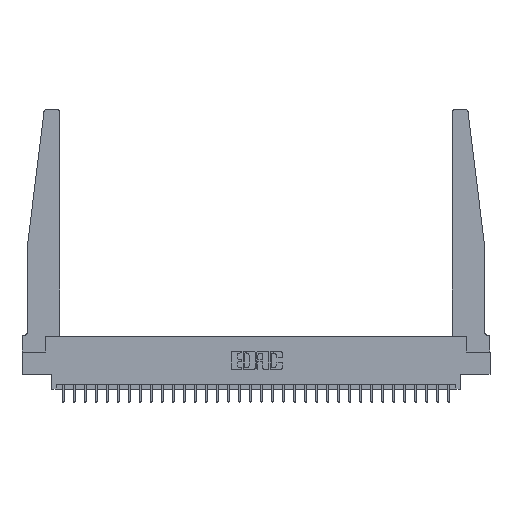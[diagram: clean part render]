
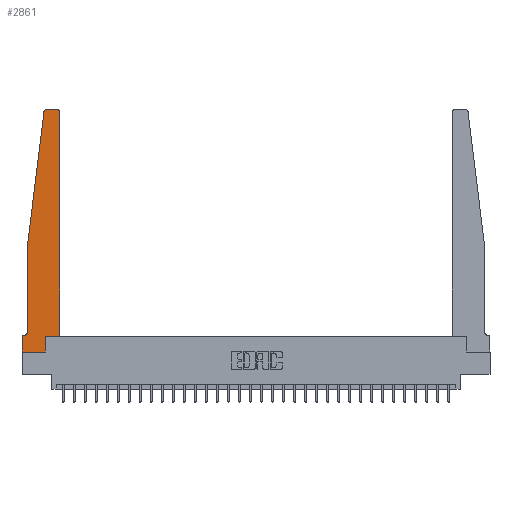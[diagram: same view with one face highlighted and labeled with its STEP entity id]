
A CAD part, top view. The second image highlights one B-rep face of the part: STEP entity #2861.
In plain terms, the highlighted planar face has unit normal (0, 0, 1).
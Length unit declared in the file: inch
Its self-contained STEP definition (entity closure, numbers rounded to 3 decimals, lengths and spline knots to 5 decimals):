
#113 = VECTOR ( 'NONE', #15878, 39.37008 ) ;
#604 = VECTOR ( 'NONE', #16311, 39.37008 ) ;
#1210 = CARTESIAN_POINT ( 'NONE',  ( 0., 0., 0.37 ) ) ;
#1375 = AXIS2_PLACEMENT_3D ( 'NONE', #19263, #5602, #28424 ) ;
#2114 = EDGE_CURVE ( 'NONE', #11931, #7090, #2983, .T. ) ;
#2185 = FACE_OUTER_BOUND ( 'NONE', #9583, .T. ) ;
#2272 = EDGE_CURVE ( 'NONE', #24319, #6425, #29254, .T. ) ;
#2337 = LINE ( 'NONE', #8974, #113 ) ;
#2735 = DIRECTION ( 'NONE',  ( -0.122, -0.992, 0. ) ) ;
#2861 = ADVANCED_FACE ( 'NONE', ( #2185 ), #18413, .T. ) ;
#2983 = LINE ( 'NONE', #17113, #20134 ) ;
#3776 = CARTESIAN_POINT ( 'NONE',  ( 0.2605, 0.18, 0.37 ) ) ;
#3789 = VECTOR ( 'NONE', #28690, 39.37008 ) ;
#4310 = VECTOR ( 'NONE', #5307, 39.37008 ) ;
#4669 = VERTEX_POINT ( 'NONE', #16629 ) ;
#4788 = VERTEX_POINT ( 'NONE', #5930 ) ;
#5070 = CARTESIAN_POINT ( 'NONE',  ( 0.015, 0.1875, 0.37 ) ) ;
#5114 = ORIENTED_EDGE ( 'NONE', *, *, #6896, .T. ) ;
#5252 = DIRECTION ( 'NONE',  ( -1., 0., 0. ) ) ;
#5307 = DIRECTION ( 'NONE',  ( 1., 0., 0. ) ) ;
#5602 = DIRECTION ( 'NONE',  ( 0., 0., 1. ) ) ;
#5633 = AXIS2_PLACEMENT_3D ( 'NONE', #13264, #6187, #24934 ) ;
#5685 = ORIENTED_EDGE ( 'NONE', *, *, #8064, .T. ) ;
#5769 = EDGE_CURVE ( 'NONE', #4788, #20493, #21956, .T. ) ;
#5930 = CARTESIAN_POINT ( 'NONE',  ( 0.065, 0.2375, 0.37 ) ) ;
#6187 = DIRECTION ( 'NONE',  ( 0., 0., 1. ) ) ;
#6311 = LINE ( 'NONE', #3776, #17453 ) ;
#6425 = VERTEX_POINT ( 'NONE', #28868 ) ;
#6426 = CARTESIAN_POINT ( 'NONE',  ( 0.425, 2.72, 0.37 ) ) ;
#6454 = EDGE_CURVE ( 'NONE', #7090, #4669, #19595, .T. ) ;
#6896 = EDGE_CURVE ( 'NONE', #6425, #22124, #23873, .T. ) ;
#7037 = ORIENTED_EDGE ( 'NONE', *, *, #26764, .T. ) ;
#7060 = CARTESIAN_POINT ( 'NONE',  ( 0.27653, 2.75, 0.37 ) ) ;
#7090 = VERTEX_POINT ( 'NONE', #7060 ) ;
#7146 = ORIENTED_EDGE ( 'NONE', *, *, #17916, .T. ) ;
#7195 = DIRECTION ( 'NONE',  ( 1., 0., 0. ) ) ;
#8064 = EDGE_CURVE ( 'NONE', #26321, #11385, #9858, .T. ) ;
#8168 = CARTESIAN_POINT ( 'NONE',  ( 0., 0.1875, 0.37 ) ) ;
#8697 = CARTESIAN_POINT ( 'NONE',  ( 0.425, 0.18, 0.37 ) ) ;
#8974 = CARTESIAN_POINT ( 'NONE',  ( 0.065, 1.25, 0.37 ) ) ;
#9503 = CIRCLE ( 'NONE', #5633, 0.03 ) ;
#9583 = EDGE_LOOP ( 'NONE', ( #20952, #18954, #13640, #7146, #17801, #12835, #13580, #5685, #7037, #19725, #5114, #25867 ) ) ;
#9858 = LINE ( 'NONE', #28140, #4310 ) ;
#10112 = LINE ( 'NONE', #1210, #13835 ) ;
#10404 = CARTESIAN_POINT ( 'NONE',  ( 0.425, 0.18, 0.37 ) ) ;
#11379 = DIRECTION ( 'NONE',  ( 1., 0., 0. ) ) ;
#11385 = VERTEX_POINT ( 'NONE', #22974 ) ;
#11838 = CARTESIAN_POINT ( 'NONE',  ( 0.015, 0.2375, 0.37 ) ) ;
#11931 = VERTEX_POINT ( 'NONE', #12268 ) ;
#11979 = DIRECTION ( 'NONE',  ( 0., 0., -1. ) ) ;
#12268 = CARTESIAN_POINT ( 'NONE',  ( 0.395, 2.75, 0.37 ) ) ;
#12835 = ORIENTED_EDGE ( 'NONE', *, *, #18212, .T. ) ;
#13264 = CARTESIAN_POINT ( 'NONE',  ( 0.395, 2.72, 0.37 ) ) ;
#13580 = ORIENTED_EDGE ( 'NONE', *, *, #14217, .T. ) ;
#13640 = ORIENTED_EDGE ( 'NONE', *, *, #21345, .T. ) ;
#13835 = VECTOR ( 'NONE', #23576, 39.37008 ) ;
#13854 = VERTEX_POINT ( 'NONE', #15510 ) ;
#13889 = EDGE_CURVE ( 'NONE', #22124, #11931, #9503, .T. ) ;
#14070 = DIRECTION ( 'NONE',  ( -1., 0., 0. ) ) ;
#14217 = EDGE_CURVE ( 'NONE', #22931, #26321, #10112, .T. ) ;
#14469 = LINE ( 'NONE', #23308, #29025 ) ;
#15510 = CARTESIAN_POINT ( 'NONE',  ( 0.065, 1.25, 0.37 ) ) ;
#15878 = DIRECTION ( 'NONE',  ( 0., -1., 0. ) ) ;
#16311 = DIRECTION ( 'NONE',  ( -1., 0., 0. ) ) ;
#16456 = CARTESIAN_POINT ( 'NONE',  ( 0.065, 0.1875, 0.37 ) ) ;
#16629 = CARTESIAN_POINT ( 'NONE',  ( 0.24675, 2.72367, 0.37 ) ) ;
#16751 = LINE ( 'NONE', #16456, #604 ) ;
#17113 = CARTESIAN_POINT ( 'NONE',  ( 0.25, 2.75, 0.37 ) ) ;
#17453 = VECTOR ( 'NONE', #19395, 39.37008 ) ;
#17801 = ORIENTED_EDGE ( 'NONE', *, *, #5769, .T. ) ;
#17916 = EDGE_CURVE ( 'NONE', #13854, #4788, #2337, .T. ) ;
#18117 = DIRECTION ( 'NONE',  ( 0., 0., 1. ) ) ;
#18212 = EDGE_CURVE ( 'NONE', #20493, #22931, #16751, .T. ) ;
#18413 = PLANE ( 'NONE',  #19465 ) ;
#18480 = VECTOR ( 'NONE', #7195, 39.37008 ) ;
#18954 = ORIENTED_EDGE ( 'NONE', *, *, #6454, .T. ) ;
#19081 = AXIS2_PLACEMENT_3D ( 'NONE', #11838, #11979, #14070 ) ;
#19263 = CARTESIAN_POINT ( 'NONE',  ( 0.27653, 2.72, 0.37 ) ) ;
#19395 = DIRECTION ( 'NONE',  ( 0., 1., 0. ) ) ;
#19465 = AXIS2_PLACEMENT_3D ( 'NONE', #27553, #18117, #11379 ) ;
#19595 = CIRCLE ( 'NONE', #1375, 0.03 ) ;
#19620 = CARTESIAN_POINT ( 'NONE',  ( 0., 0., 0.37 ) ) ;
#19725 = ORIENTED_EDGE ( 'NONE', *, *, #2272, .T. ) ;
#20134 = VECTOR ( 'NONE', #5252, 39.37008 ) ;
#20493 = VERTEX_POINT ( 'NONE', #5070 ) ;
#20952 = ORIENTED_EDGE ( 'NONE', *, *, #2114, .T. ) ;
#21345 = EDGE_CURVE ( 'NONE', #4669, #13854, #14469, .T. ) ;
#21956 = CIRCLE ( 'NONE', #19081, 0.05 ) ;
#22124 = VERTEX_POINT ( 'NONE', #6426 ) ;
#22931 = VERTEX_POINT ( 'NONE', #8168 ) ;
#22974 = CARTESIAN_POINT ( 'NONE',  ( 0.2605, 0., 0.37 ) ) ;
#23308 = CARTESIAN_POINT ( 'NONE',  ( 0.065, 1.25, 0.37 ) ) ;
#23576 = DIRECTION ( 'NONE',  ( 0., -1., 0. ) ) ;
#23873 = LINE ( 'NONE', #10404, #3789 ) ;
#24319 = VERTEX_POINT ( 'NONE', #28318 ) ;
#24934 = DIRECTION ( 'NONE',  ( 1., 0., 0. ) ) ;
#25867 = ORIENTED_EDGE ( 'NONE', *, *, #13889, .T. ) ;
#26321 = VERTEX_POINT ( 'NONE', #19620 ) ;
#26764 = EDGE_CURVE ( 'NONE', #11385, #24319, #6311, .T. ) ;
#27553 = CARTESIAN_POINT ( 'NONE',  ( 0., 0.1875, 0.37 ) ) ;
#28140 = CARTESIAN_POINT ( 'NONE',  ( 0., 0., 0.37 ) ) ;
#28318 = CARTESIAN_POINT ( 'NONE',  ( 0.2605, 0.18, 0.37 ) ) ;
#28424 = DIRECTION ( 'NONE',  ( 1., 0., 0. ) ) ;
#28690 = DIRECTION ( 'NONE',  ( 0., 1., 0. ) ) ;
#28868 = CARTESIAN_POINT ( 'NONE',  ( 0.425, 0.18, 0.37 ) ) ;
#29025 = VECTOR ( 'NONE', #2735, 39.37008 ) ;
#29254 = LINE ( 'NONE', #8697, #18480 ) ;
